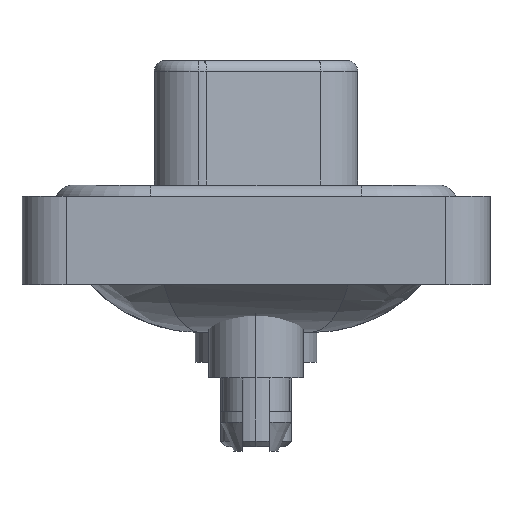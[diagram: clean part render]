
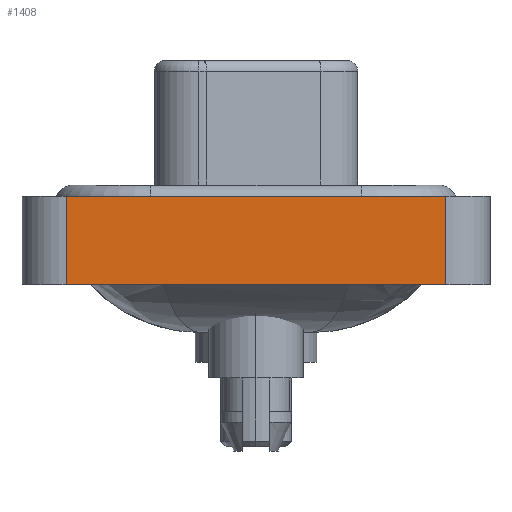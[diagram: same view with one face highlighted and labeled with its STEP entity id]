
A CAD part, left-side view. The second image highlights one B-rep face of the part: STEP entity #1408.
In plain terms, the highlighted planar face has unit normal (-1, 0, 0).
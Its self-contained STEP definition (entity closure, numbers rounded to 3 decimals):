
#31 = ORIENTED_EDGE ( 'NONE', *, *, #10380, .F. ) ;
#886 = CARTESIAN_POINT ( 'NONE',  ( -7.35, -8.55, -3.6 ) ) ;
#1081 = DIRECTION ( 'NONE',  ( 0., 0., 1. ) ) ;
#1404 = LINE ( 'NONE', #8837, #9512 ) ;
#1408 = ADVANCED_FACE ( 'NONE', ( #9359 ), #14124, .T. ) ;
#5083 = LINE ( 'NONE', #6842, #20086 ) ;
#5357 = VERTEX_POINT ( 'NONE', #886 ) ;
#5846 = CARTESIAN_POINT ( 'NONE',  ( -7.35, -8.55, 0.4 ) ) ;
#6374 = VERTEX_POINT ( 'NONE', #18563 ) ;
#6842 = CARTESIAN_POINT ( 'NONE',  ( -7.35, -8.55, -3.6 ) ) ;
#6875 = DIRECTION ( 'NONE',  ( 0., 0., 1. ) ) ;
#8453 = EDGE_LOOP ( 'NONE', ( #10777, #31, #21904, #14434 ) ) ;
#8676 = CARTESIAN_POINT ( 'NONE',  ( -7.35, 8.55, 0.4 ) ) ;
#8837 = CARTESIAN_POINT ( 'NONE',  ( -7.35, 8.55, -3.6 ) ) ;
#9359 = FACE_OUTER_BOUND ( 'NONE', #8453, .T. ) ;
#9512 = VECTOR ( 'NONE', #6875, 1000. ) ;
#9838 = DIRECTION ( 'NONE',  ( 0., -1., 0. ) ) ;
#10380 = EDGE_CURVE ( 'NONE', #17659, #19226, #21722, .T. ) ;
#10777 = ORIENTED_EDGE ( 'NONE', *, *, #19105, .T. ) ;
#11517 = CARTESIAN_POINT ( 'NONE',  ( -7.35, -8.55, -3.6 ) ) ;
#13060 = VECTOR ( 'NONE', #1081, 1000. ) ;
#14124 = PLANE ( 'NONE',  #17246 ) ;
#14434 = ORIENTED_EDGE ( 'NONE', *, *, #18074, .T. ) ;
#14570 = DIRECTION ( 'NONE',  ( 0., 0., 1. ) ) ;
#15115 = LINE ( 'NONE', #11517, #13060 ) ;
#16275 = DIRECTION ( 'NONE',  ( 0., -1., 0. ) ) ;
#16506 = VECTOR ( 'NONE', #16275, 1000. ) ;
#17246 = AXIS2_PLACEMENT_3D ( 'NONE', #19690, #21337, #14570 ) ;
#17659 = VERTEX_POINT ( 'NONE', #8676 ) ;
#18074 = EDGE_CURVE ( 'NONE', #6374, #5357, #5083, .T. ) ;
#18563 = CARTESIAN_POINT ( 'NONE',  ( -7.35, 8.55, -3.6 ) ) ;
#19105 = EDGE_CURVE ( 'NONE', #5357, #19226, #15115, .T. ) ;
#19226 = VERTEX_POINT ( 'NONE', #22799 ) ;
#19690 = CARTESIAN_POINT ( 'NONE',  ( -7.35, -8.55, -3.6 ) ) ;
#20086 = VECTOR ( 'NONE', #9838, 1000. ) ;
#20993 = EDGE_CURVE ( 'NONE', #6374, #17659, #1404, .T. ) ;
#21337 = DIRECTION ( 'NONE',  ( -1., 0., 0. ) ) ;
#21722 = LINE ( 'NONE', #5846, #16506 ) ;
#21904 = ORIENTED_EDGE ( 'NONE', *, *, #20993, .F. ) ;
#22799 = CARTESIAN_POINT ( 'NONE',  ( -7.35, -8.55, 0.4 ) ) ;
